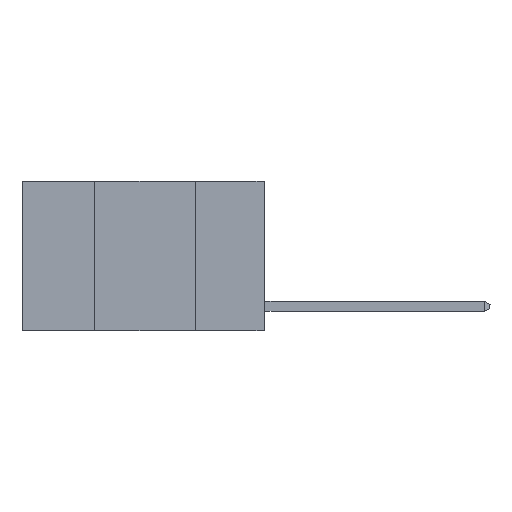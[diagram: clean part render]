
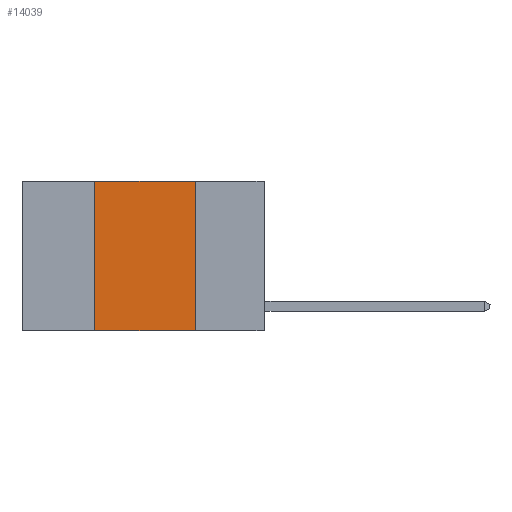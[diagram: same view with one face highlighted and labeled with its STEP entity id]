
A CAD part, left-side view. The second image highlights one B-rep face of the part: STEP entity #14039.
In plain terms, the highlighted planar face has unit normal (-1, 0, 0).
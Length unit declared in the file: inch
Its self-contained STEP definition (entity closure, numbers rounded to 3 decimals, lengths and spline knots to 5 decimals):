
#70 = VECTOR ( 'NONE', #5337, 39.37008 ) ;
#109 = CARTESIAN_POINT ( 'NONE',  ( 0., 0.6, -0.37 ) ) ;
#192 = LINE ( 'NONE', #109, #70 ) ;
#284 = PLANE ( 'NONE',  #12007 ) ;
#719 = CARTESIAN_POINT ( 'NONE',  ( 0., 0.17, 0. ) ) ;
#1084 = EDGE_CURVE ( 'NONE', #9024, #15772, #13295, .T. ) ;
#1211 = DIRECTION ( 'NONE',  ( 1., 0., 0. ) ) ;
#1514 = CARTESIAN_POINT ( 'NONE',  ( 0., 0.6, 0. ) ) ;
#2311 = DIRECTION ( 'NONE',  ( 0., 0., -1. ) ) ;
#3547 = ORIENTED_EDGE ( 'NONE', *, *, #1084, .F. ) ;
#3727 = EDGE_CURVE ( 'NONE', #15772, #14297, #14771, .T. ) ;
#4144 = EDGE_CURVE ( 'NONE', #13110, #14297, #192, .T. ) ;
#5337 = DIRECTION ( 'NONE',  ( 0., -1., 0. ) ) ;
#5405 = CARTESIAN_POINT ( 'NONE',  ( 0., 0.17, -0.37 ) ) ;
#6309 = EDGE_CURVE ( 'NONE', #13110, #9024, #9430, .T. ) ;
#6706 = DIRECTION ( 'NONE',  ( 0., 0., 1. ) ) ;
#6786 = CARTESIAN_POINT ( 'NONE',  ( 0., 0.6, 0. ) ) ;
#7270 = EDGE_LOOP ( 'NONE', ( #16788, #3547, #15264, #9356 ) ) ;
#7315 = CARTESIAN_POINT ( 'NONE',  ( 0., 0.42, 0. ) ) ;
#9024 = VERTEX_POINT ( 'NONE', #7315 ) ;
#9356 = ORIENTED_EDGE ( 'NONE', *, *, #4144, .T. ) ;
#9430 = LINE ( 'NONE', #15713, #10209 ) ;
#9794 = CARTESIAN_POINT ( 'NONE',  ( 0., 0.17, 0. ) ) ;
#10209 = VECTOR ( 'NONE', #6706, 39.37008 ) ;
#10794 = CARTESIAN_POINT ( 'NONE',  ( 0., 0.42, -0.37 ) ) ;
#10999 = VECTOR ( 'NONE', #15196, 39.37008 ) ;
#12006 = DIRECTION ( 'NONE',  ( 0., -1., 0. ) ) ;
#12007 = AXIS2_PLACEMENT_3D ( 'NONE', #1514, #1211, #2311 ) ;
#13110 = VERTEX_POINT ( 'NONE', #10794 ) ;
#13295 = LINE ( 'NONE', #6786, #13698 ) ;
#13698 = VECTOR ( 'NONE', #12006, 39.37008 ) ;
#14039 = ADVANCED_FACE ( 'NONE', ( #16458 ), #284, .F. ) ;
#14297 = VERTEX_POINT ( 'NONE', #5405 ) ;
#14771 = LINE ( 'NONE', #719, #10999 ) ;
#15196 = DIRECTION ( 'NONE',  ( 0., 0., -1. ) ) ;
#15264 = ORIENTED_EDGE ( 'NONE', *, *, #6309, .F. ) ;
#15713 = CARTESIAN_POINT ( 'NONE',  ( 0., 0.42, 0. ) ) ;
#15772 = VERTEX_POINT ( 'NONE', #9794 ) ;
#16458 = FACE_OUTER_BOUND ( 'NONE', #7270, .T. ) ;
#16788 = ORIENTED_EDGE ( 'NONE', *, *, #3727, .F. ) ;
